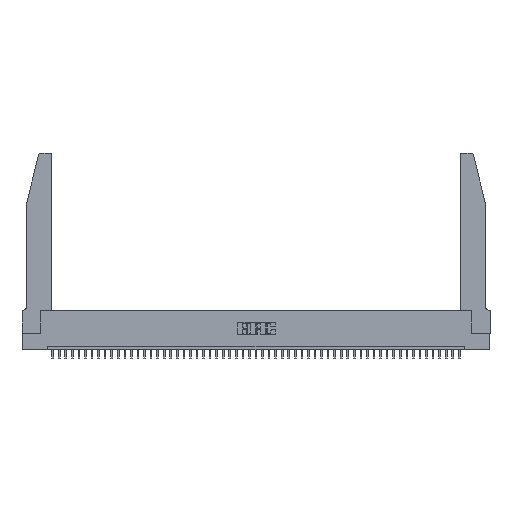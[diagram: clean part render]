
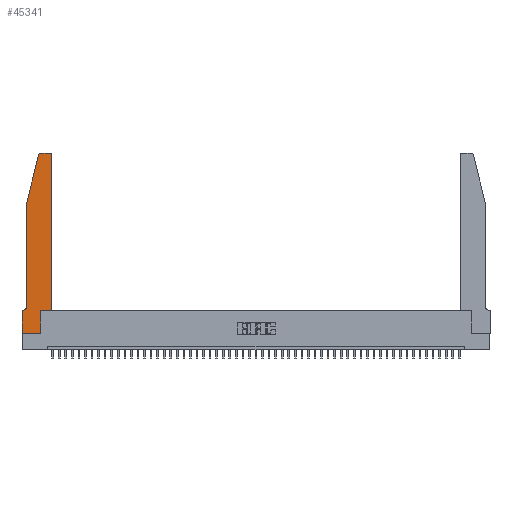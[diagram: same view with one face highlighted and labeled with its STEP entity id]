
A CAD part, top view. The second image highlights one B-rep face of the part: STEP entity #45341.
In plain terms, the highlighted planar face has unit normal (0, 0, 1).
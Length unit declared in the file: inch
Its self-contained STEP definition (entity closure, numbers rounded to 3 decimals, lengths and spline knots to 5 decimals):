
#137 = EDGE_CURVE ( 'NONE', #813, #36795, #36883, .T. ) ;
#275 = VECTOR ( 'NONE', #27324, 39.37008 ) ;
#813 = VERTEX_POINT ( 'NONE', #39266 ) ;
#844 = EDGE_CURVE ( 'NONE', #39866, #4873, #27239, .T. ) ;
#3037 = EDGE_CURVE ( 'NONE', #25649, #27027, #47915, .T. ) ;
#3056 = ORIENTED_EDGE ( 'NONE', *, *, #11592, .T. ) ;
#3089 = CARTESIAN_POINT ( 'NONE',  ( 0.25487, 2.72718, 0.37 ) ) ;
#3464 = DIRECTION ( 'NONE',  ( -1., 0., 0. ) ) ;
#4202 = ORIENTED_EDGE ( 'NONE', *, *, #33785, .T. ) ;
#4420 = EDGE_CURVE ( 'NONE', #27027, #48986, #34361, .T. ) ;
#4873 = VERTEX_POINT ( 'NONE', #15056 ) ;
#5118 = ORIENTED_EDGE ( 'NONE', *, *, #15716, .T. ) ;
#5707 = DIRECTION ( 'NONE',  ( 1., 0., 0. ) ) ;
#6320 = VECTOR ( 'NONE', #46060, 39.37008 ) ;
#7571 = CIRCLE ( 'NONE', #46094, 0.03 ) ;
#7647 = LINE ( 'NONE', #35396, #24320 ) ;
#8002 = CARTESIAN_POINT ( 'NONE',  ( 0.4505, 2.72, 0.37 ) ) ;
#8667 = CIRCLE ( 'NONE', #32432, 0.03 ) ;
#8882 = CARTESIAN_POINT ( 'NONE',  ( 0., 0., 0.37 ) ) ;
#8948 = CARTESIAN_POINT ( 'NONE',  ( 0.284, 2.72, 0.37 ) ) ;
#9065 = LINE ( 'NONE', #19525, #25190 ) ;
#9526 = VERTEX_POINT ( 'NONE', #41384 ) ;
#11592 = EDGE_CURVE ( 'NONE', #48986, #48953, #7647, .T. ) ;
#12613 = EDGE_CURVE ( 'NONE', #9526, #29462, #21255, .T. ) ;
#12727 = EDGE_CURVE ( 'NONE', #21774, #39866, #8667, .T. ) ;
#12763 = DIRECTION ( 'NONE',  ( 0., 0., 1. ) ) ;
#13596 = DIRECTION ( 'NONE',  ( 0., -1., 0. ) ) ;
#15056 = CARTESIAN_POINT ( 'NONE',  ( 0.0755, 2., 0.37 ) ) ;
#15716 = EDGE_CURVE ( 'NONE', #4873, #25649, #40671, .T. ) ;
#15833 = DIRECTION ( 'NONE',  ( 1., 0., 0. ) ) ;
#16693 = LINE ( 'NONE', #19358, #36361 ) ;
#16950 = CARTESIAN_POINT ( 'NONE',  ( 0.0755, 0.42, 0.37 ) ) ;
#17462 = DIRECTION ( 'NONE',  ( 1., 0., 0. ) ) ;
#17537 = CARTESIAN_POINT ( 'NONE',  ( 0.284, 2.75, 0.37 ) ) ;
#17803 = VECTOR ( 'NONE', #44232, 39.37008 ) ;
#18667 = DIRECTION ( 'NONE',  ( 1., 0., 0. ) ) ;
#19000 = DIRECTION ( 'NONE',  ( 0., 0., -1. ) ) ;
#19358 = CARTESIAN_POINT ( 'NONE',  ( 0.2605, 2.75, 0.37 ) ) ;
#19525 = CARTESIAN_POINT ( 'NONE',  ( 0., 0., 0.37 ) ) ;
#19925 = CARTESIAN_POINT ( 'NONE',  ( 0.2865, 0.35, 0.37 ) ) ;
#20484 = LINE ( 'NONE', #33177, #41964 ) ;
#21255 = LINE ( 'NONE', #40384, #275 ) ;
#21323 = DIRECTION ( 'NONE',  ( 0., 0., 1. ) ) ;
#21739 = ORIENTED_EDGE ( 'NONE', *, *, #25390, .T. ) ;
#21774 = VERTEX_POINT ( 'NONE', #17537 ) ;
#23306 = DIRECTION ( 'NONE',  ( -0.239, -0.971, 0. ) ) ;
#23575 = EDGE_CURVE ( 'NONE', #29462, #29763, #7571, .T. ) ;
#24320 = VECTOR ( 'NONE', #31749, 39.37008 ) ;
#25190 = VECTOR ( 'NONE', #15833, 39.37008 ) ;
#25390 = EDGE_CURVE ( 'NONE', #36795, #9526, #20484, .T. ) ;
#25649 = VERTEX_POINT ( 'NONE', #16950 ) ;
#27027 = VERTEX_POINT ( 'NONE', #36267 ) ;
#27239 = LINE ( 'NONE', #43108, #46846 ) ;
#27324 = DIRECTION ( 'NONE',  ( 0., 1., 0. ) ) ;
#28275 = CARTESIAN_POINT ( 'NONE',  ( 0., 0.35, 0.37 ) ) ;
#28733 = AXIS2_PLACEMENT_3D ( 'NONE', #28275, #21323, #17462 ) ;
#29332 = ORIENTED_EDGE ( 'NONE', *, *, #3037, .T. ) ;
#29462 = VERTEX_POINT ( 'NONE', #8002 ) ;
#29468 = FACE_OUTER_BOUND ( 'NONE', #46426, .T. ) ;
#29763 = VERTEX_POINT ( 'NONE', #36819 ) ;
#29858 = ORIENTED_EDGE ( 'NONE', *, *, #39674, .T. ) ;
#30535 = VECTOR ( 'NONE', #13596, 39.37008 ) ;
#30640 = AXIS2_PLACEMENT_3D ( 'NONE', #41835, #19000, #3464 ) ;
#31749 = DIRECTION ( 'NONE',  ( 0., -1., 0. ) ) ;
#32432 = AXIS2_PLACEMENT_3D ( 'NONE', #8948, #12763, #39411 ) ;
#32581 = CARTESIAN_POINT ( 'NONE',  ( 0.2865, 0.35, 0.37 ) ) ;
#32617 = CARTESIAN_POINT ( 'NONE',  ( 0.0755, 2., 0.37 ) ) ;
#33177 = CARTESIAN_POINT ( 'NONE',  ( 0.4505, 0.35, 0.37 ) ) ;
#33785 = EDGE_CURVE ( 'NONE', #29763, #21774, #16693, .T. ) ;
#34361 = LINE ( 'NONE', #45766, #6320 ) ;
#35281 = ORIENTED_EDGE ( 'NONE', *, *, #23575, .T. ) ;
#35396 = CARTESIAN_POINT ( 'NONE',  ( 0., 0., 0.37 ) ) ;
#36267 = CARTESIAN_POINT ( 'NONE',  ( 0.0055, 0.35, 0.37 ) ) ;
#36361 = VECTOR ( 'NONE', #45977, 39.37008 ) ;
#36795 = VERTEX_POINT ( 'NONE', #19925 ) ;
#36819 = CARTESIAN_POINT ( 'NONE',  ( 0.4205, 2.75, 0.37 ) ) ;
#36883 = LINE ( 'NONE', #32581, #17803 ) ;
#38084 = ORIENTED_EDGE ( 'NONE', *, *, #12613, .T. ) ;
#38574 = ORIENTED_EDGE ( 'NONE', *, *, #137, .T. ) ;
#39008 = ORIENTED_EDGE ( 'NONE', *, *, #4420, .T. ) ;
#39091 = CARTESIAN_POINT ( 'NONE',  ( 0.4205, 2.72, 0.37 ) ) ;
#39266 = CARTESIAN_POINT ( 'NONE',  ( 0.2865, 0., 0.37 ) ) ;
#39411 = DIRECTION ( 'NONE',  ( 1., 0., 0. ) ) ;
#39528 = CARTESIAN_POINT ( 'NONE',  ( 0., 0.35, 0.37 ) ) ;
#39674 = EDGE_CURVE ( 'NONE', #48953, #813, #9065, .T. ) ;
#39866 = VERTEX_POINT ( 'NONE', #3089 ) ;
#40076 = ORIENTED_EDGE ( 'NONE', *, *, #12727, .T. ) ;
#40244 = ORIENTED_EDGE ( 'NONE', *, *, #844, .T. ) ;
#40384 = CARTESIAN_POINT ( 'NONE',  ( 0.4505, 0.35, 0.37 ) ) ;
#40671 = LINE ( 'NONE', #32617, #30535 ) ;
#41384 = CARTESIAN_POINT ( 'NONE',  ( 0.4505, 0.35, 0.37 ) ) ;
#41835 = CARTESIAN_POINT ( 'NONE',  ( 0.0055, 0.42, 0.37 ) ) ;
#41964 = VECTOR ( 'NONE', #18667, 39.37008 ) ;
#43108 = CARTESIAN_POINT ( 'NONE',  ( 0.0755, 2., 0.37 ) ) ;
#44232 = DIRECTION ( 'NONE',  ( 0., 1., 0. ) ) ;
#45341 = ADVANCED_FACE ( 'NONE', ( #29468 ), #47763, .T. ) ;
#45766 = CARTESIAN_POINT ( 'NONE',  ( 0.0755, 0.35, 0.37 ) ) ;
#45977 = DIRECTION ( 'NONE',  ( -1., 0., 0. ) ) ;
#46060 = DIRECTION ( 'NONE',  ( -1., 0., 0. ) ) ;
#46094 = AXIS2_PLACEMENT_3D ( 'NONE', #39091, #47545, #5707 ) ;
#46426 = EDGE_LOOP ( 'NONE', ( #4202, #40076, #40244, #5118, #29332, #39008, #3056, #29858, #38574, #21739, #38084, #35281 ) ) ;
#46846 = VECTOR ( 'NONE', #23306, 39.37008 ) ;
#47545 = DIRECTION ( 'NONE',  ( 0., 0., 1. ) ) ;
#47763 = PLANE ( 'NONE',  #28733 ) ;
#47915 = CIRCLE ( 'NONE', #30640, 0.07 ) ;
#48953 = VERTEX_POINT ( 'NONE', #8882 ) ;
#48986 = VERTEX_POINT ( 'NONE', #39528 ) ;
